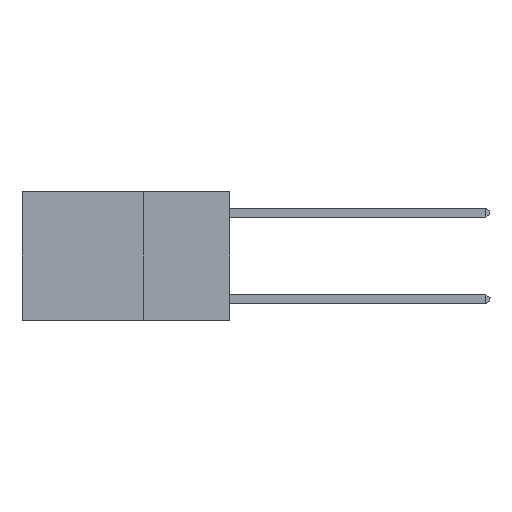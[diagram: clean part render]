
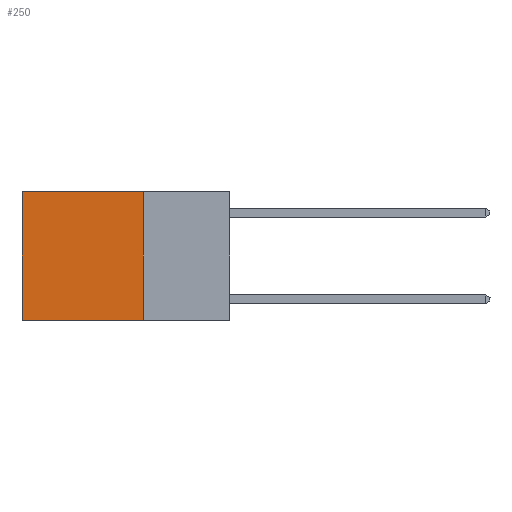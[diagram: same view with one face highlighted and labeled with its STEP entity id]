
A CAD part, left-side view. The second image highlights one B-rep face of the part: STEP entity #250.
In plain terms, the highlighted planar face has unit normal (-1, 0, 0).
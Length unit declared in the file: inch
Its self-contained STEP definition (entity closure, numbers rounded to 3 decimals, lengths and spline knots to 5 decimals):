
#187 = DIRECTION ( 'NONE',  ( 0., 0., -1. ) ) ;
#223 = VECTOR ( 'NONE', #16265, 39.37008 ) ;
#250 = ADVANCED_FACE ( 'NONE', ( #7567 ), #8109, .F. ) ;
#381 = DIRECTION ( 'NONE',  ( 0., 1., 0. ) ) ;
#1265 = CARTESIAN_POINT ( 'NONE',  ( 0.2625, 0.6, 0. ) ) ;
#1326 = AXIS2_PLACEMENT_3D ( 'NONE', #8211, #7997, #7951 ) ;
#1953 = VECTOR ( 'NONE', #187, 39.37008 ) ;
#2241 = VERTEX_POINT ( 'NONE', #1265 ) ;
#2536 = ORIENTED_EDGE ( 'NONE', *, *, #12941, .F. ) ;
#2749 = VERTEX_POINT ( 'NONE', #9283 ) ;
#2963 = VERTEX_POINT ( 'NONE', #8173 ) ;
#2998 = CARTESIAN_POINT ( 'NONE',  ( 0.2625, 0.25, -0.37 ) ) ;
#3754 = ORIENTED_EDGE ( 'NONE', *, *, #14716, .T. ) ;
#5425 = DIRECTION ( 'NONE',  ( 0., 0., -1. ) ) ;
#5970 = LINE ( 'NONE', #10342, #1953 ) ;
#6005 = EDGE_LOOP ( 'NONE', ( #10486, #2536, #18372, #3754 ) ) ;
#6862 = EDGE_CURVE ( 'NONE', #2749, #14971, #5970, .T. ) ;
#6917 = EDGE_CURVE ( 'NONE', #2241, #2963, #18788, .T. ) ;
#7344 = LINE ( 'NONE', #8864, #11272 ) ;
#7567 = FACE_OUTER_BOUND ( 'NONE', #6005, .T. ) ;
#7951 = DIRECTION ( 'NONE',  ( 0., 0., -1. ) ) ;
#7997 = DIRECTION ( 'NONE',  ( 1., 0., 0. ) ) ;
#8109 = PLANE ( 'NONE',  #1326 ) ;
#8173 = CARTESIAN_POINT ( 'NONE',  ( 0.2625, 0.6, -0.37 ) ) ;
#8211 = CARTESIAN_POINT ( 'NONE',  ( 0.2625, 0.25, 0. ) ) ;
#8864 = CARTESIAN_POINT ( 'NONE',  ( 0.2625, 0.25, 0. ) ) ;
#9283 = CARTESIAN_POINT ( 'NONE',  ( 0.2625, 0.25, 0. ) ) ;
#9918 = VECTOR ( 'NONE', #5425, 39.37008 ) ;
#10342 = CARTESIAN_POINT ( 'NONE',  ( 0.2625, 0.25, 0. ) ) ;
#10486 = ORIENTED_EDGE ( 'NONE', *, *, #6917, .T. ) ;
#11272 = VECTOR ( 'NONE', #381, 39.37008 ) ;
#12815 = CARTESIAN_POINT ( 'NONE',  ( 0.2625, 0.25, -0.37 ) ) ;
#12941 = EDGE_CURVE ( 'NONE', #14971, #2963, #18138, .T. ) ;
#14716 = EDGE_CURVE ( 'NONE', #2749, #2241, #7344, .T. ) ;
#14971 = VERTEX_POINT ( 'NONE', #12815 ) ;
#16265 = DIRECTION ( 'NONE',  ( 0., 1., 0. ) ) ;
#17121 = CARTESIAN_POINT ( 'NONE',  ( 0.2625, 0.6, 0. ) ) ;
#18138 = LINE ( 'NONE', #2998, #223 ) ;
#18372 = ORIENTED_EDGE ( 'NONE', *, *, #6862, .F. ) ;
#18788 = LINE ( 'NONE', #17121, #9918 ) ;
